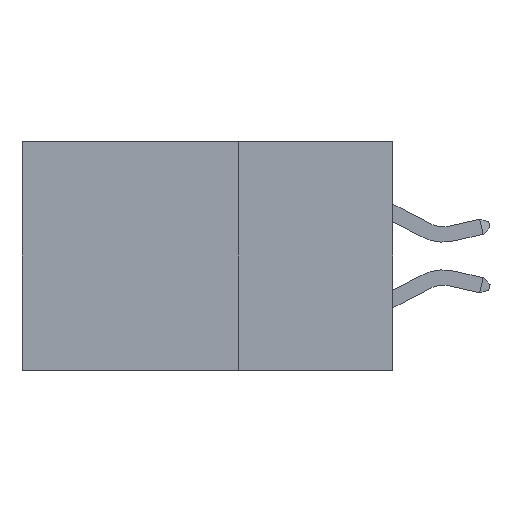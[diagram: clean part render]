
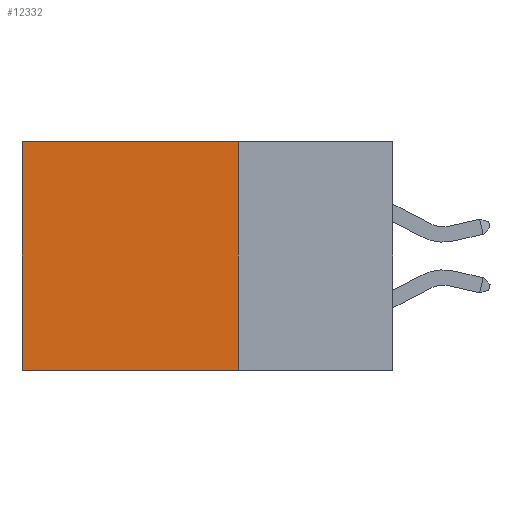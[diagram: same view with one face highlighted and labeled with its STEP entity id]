
A CAD part, left-side view. The second image highlights one B-rep face of the part: STEP entity #12332.
In plain terms, the highlighted planar face has unit normal (-1, 0, 0).
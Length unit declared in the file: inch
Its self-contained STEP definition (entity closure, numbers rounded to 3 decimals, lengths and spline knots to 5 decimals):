
#580 = VERTEX_POINT ( 'NONE', #9147 ) ;
#810 = DIRECTION ( 'NONE',  ( 0., 1., 0. ) ) ;
#945 = VECTOR ( 'NONE', #11927, 39.37008 ) ;
#1222 = VECTOR ( 'NONE', #6251, 39.37008 ) ;
#1810 = AXIS2_PLACEMENT_3D ( 'NONE', #9919, #14049, #7794 ) ;
#2045 = EDGE_CURVE ( 'NONE', #580, #8164, #12937, .T. ) ;
#3307 = CARTESIAN_POINT ( 'NONE',  ( 0.2875, 0.6, 0. ) ) ;
#3387 = VECTOR ( 'NONE', #810, 39.37008 ) ;
#3413 = EDGE_LOOP ( 'NONE', ( #13488, #3514, #11238, #6968 ) ) ;
#3514 = ORIENTED_EDGE ( 'NONE', *, *, #5465, .F. ) ;
#3544 = FACE_OUTER_BOUND ( 'NONE', #3413, .T. ) ;
#4313 = LINE ( 'NONE', #11609, #1222 ) ;
#4373 = VECTOR ( 'NONE', #7977, 39.37008 ) ;
#5465 = EDGE_CURVE ( 'NONE', #7561, #13982, #6415, .T. ) ;
#6251 = DIRECTION ( 'NONE',  ( 0., 0., -1. ) ) ;
#6415 = LINE ( 'NONE', #6540, #3387 ) ;
#6540 = CARTESIAN_POINT ( 'NONE',  ( 0.2875, 0.25, -0.37 ) ) ;
#6543 = CARTESIAN_POINT ( 'NONE',  ( 0.2875, 0.6, 0. ) ) ;
#6968 = ORIENTED_EDGE ( 'NONE', *, *, #2045, .T. ) ;
#7214 = EDGE_CURVE ( 'NONE', #8164, #13982, #7376, .T. ) ;
#7376 = LINE ( 'NONE', #6543, #945 ) ;
#7561 = VERTEX_POINT ( 'NONE', #10428 ) ;
#7794 = DIRECTION ( 'NONE',  ( 0., 0., -1. ) ) ;
#7977 = DIRECTION ( 'NONE',  ( 0., 1., 0. ) ) ;
#8037 = CARTESIAN_POINT ( 'NONE',  ( 0.2875, 0.25, 0. ) ) ;
#8164 = VERTEX_POINT ( 'NONE', #3307 ) ;
#9147 = CARTESIAN_POINT ( 'NONE',  ( 0.2875, 0.25, 0. ) ) ;
#9919 = CARTESIAN_POINT ( 'NONE',  ( 0.2875, 0.25, 0. ) ) ;
#10428 = CARTESIAN_POINT ( 'NONE',  ( 0.2875, 0.25, -0.37 ) ) ;
#10985 = EDGE_CURVE ( 'NONE', #580, #7561, #4313, .T. ) ;
#11238 = ORIENTED_EDGE ( 'NONE', *, *, #10985, .F. ) ;
#11609 = CARTESIAN_POINT ( 'NONE',  ( 0.2875, 0.25, 0. ) ) ;
#11927 = DIRECTION ( 'NONE',  ( 0., 0., -1. ) ) ;
#12332 = ADVANCED_FACE ( 'NONE', ( #3544 ), #12965, .F. ) ;
#12937 = LINE ( 'NONE', #8037, #4373 ) ;
#12965 = PLANE ( 'NONE',  #1810 ) ;
#13435 = CARTESIAN_POINT ( 'NONE',  ( 0.2875, 0.6, -0.37 ) ) ;
#13488 = ORIENTED_EDGE ( 'NONE', *, *, #7214, .T. ) ;
#13982 = VERTEX_POINT ( 'NONE', #13435 ) ;
#14049 = DIRECTION ( 'NONE',  ( 1., 0., 0. ) ) ;
